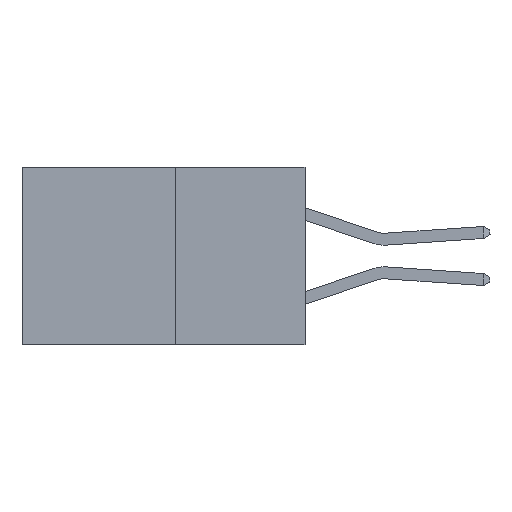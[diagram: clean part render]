
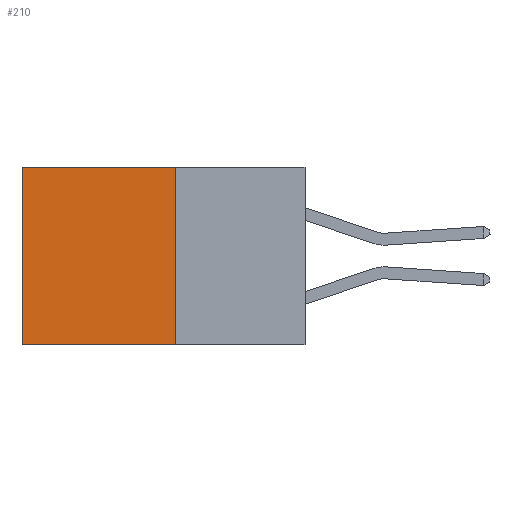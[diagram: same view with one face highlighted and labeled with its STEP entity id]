
A CAD part, left-side view. The second image highlights one B-rep face of the part: STEP entity #210.
In plain terms, the highlighted planar face has unit normal (-1, 0, 0).
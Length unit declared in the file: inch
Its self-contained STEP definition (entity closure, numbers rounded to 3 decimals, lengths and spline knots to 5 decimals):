
#95 = LINE ( 'NONE', #5107, #7827 ) ;
#210 = ADVANCED_FACE ( 'NONE', ( #955 ), #5534, .F. ) ;
#231 = CARTESIAN_POINT ( 'NONE',  ( 0.277, 0.27, -0.37 ) ) ;
#318 = ORIENTED_EDGE ( 'NONE', *, *, #6124, .T. ) ;
#370 = ORIENTED_EDGE ( 'NONE', *, *, #7153, .F. ) ;
#389 = ORIENTED_EDGE ( 'NONE', *, *, #5268, .F. ) ;
#414 = ORIENTED_EDGE ( 'NONE', *, *, #416, .T. ) ;
#416 = EDGE_CURVE ( 'NONE', #6010, #9256, #2031, .T. ) ;
#537 = LINE ( 'NONE', #4627, #4564 ) ;
#634 = DIRECTION ( 'NONE',  ( 0., 1., 0. ) ) ;
#955 = FACE_OUTER_BOUND ( 'NONE', #1270, .T. ) ;
#982 = VECTOR ( 'NONE', #5041, 39.37008 ) ;
#1151 = CARTESIAN_POINT ( 'NONE',  ( 0.277, 0.59, -0.37 ) ) ;
#1232 = DIRECTION ( 'NONE',  ( 0., 0., -1. ) ) ;
#1270 = EDGE_LOOP ( 'NONE', ( #318, #370, #389, #414 ) ) ;
#1487 = VECTOR ( 'NONE', #8944, 39.37008 ) ;
#1769 = DIRECTION ( 'NONE',  ( 1., 0., 0. ) ) ;
#2031 = LINE ( 'NONE', #9048, #1487 ) ;
#3340 = AXIS2_PLACEMENT_3D ( 'NONE', #231, #1769, #5571 ) ;
#3590 = CARTESIAN_POINT ( 'NONE',  ( 0.277, 0.59, -0.37 ) ) ;
#4564 = VECTOR ( 'NONE', #634, 39.37008 ) ;
#4627 = CARTESIAN_POINT ( 'NONE',  ( 0.277, 0.27, -0.37 ) ) ;
#5041 = DIRECTION ( 'NONE',  ( 0., 0., -1. ) ) ;
#5107 = CARTESIAN_POINT ( 'NONE',  ( 0.277, 0.27, -0.37 ) ) ;
#5117 = VERTEX_POINT ( 'NONE', #3590 ) ;
#5268 = EDGE_CURVE ( 'NONE', #6010, #6880, #95, .T. ) ;
#5534 = PLANE ( 'NONE',  #3340 ) ;
#5571 = DIRECTION ( 'NONE',  ( 0., 0., -1. ) ) ;
#6010 = VERTEX_POINT ( 'NONE', #6313 ) ;
#6124 = EDGE_CURVE ( 'NONE', #9256, #5117, #8819, .T. ) ;
#6313 = CARTESIAN_POINT ( 'NONE',  ( 0.277, 0.27, 0. ) ) ;
#6880 = VERTEX_POINT ( 'NONE', #9071 ) ;
#7153 = EDGE_CURVE ( 'NONE', #6880, #5117, #537, .T. ) ;
#7312 = CARTESIAN_POINT ( 'NONE',  ( 0.277, 0.59, 0. ) ) ;
#7827 = VECTOR ( 'NONE', #1232, 39.37008 ) ;
#8819 = LINE ( 'NONE', #1151, #982 ) ;
#8944 = DIRECTION ( 'NONE',  ( 0., 1., 0. ) ) ;
#9048 = CARTESIAN_POINT ( 'NONE',  ( 0.277, 0.27, 0. ) ) ;
#9071 = CARTESIAN_POINT ( 'NONE',  ( 0.277, 0.27, -0.37 ) ) ;
#9256 = VERTEX_POINT ( 'NONE', #7312 ) ;
